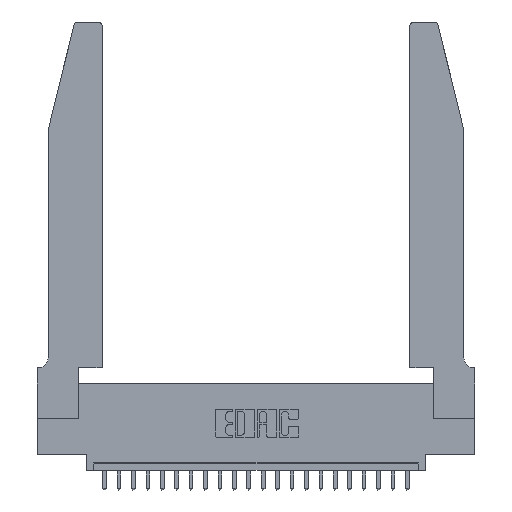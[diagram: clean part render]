
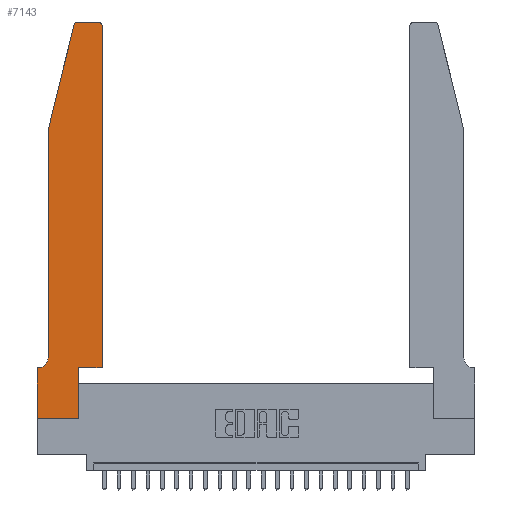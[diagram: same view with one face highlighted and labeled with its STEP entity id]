
A CAD part, top view. The second image highlights one B-rep face of the part: STEP entity #7143.
In plain terms, the highlighted planar face has unit normal (0, 0, 1).
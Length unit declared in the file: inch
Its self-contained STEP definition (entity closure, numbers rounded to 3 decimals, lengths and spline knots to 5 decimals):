
#293 = DIRECTION ( 'NONE',  ( -1., 0., 0. ) ) ;
#314 = FACE_OUTER_BOUND ( 'NONE', #9441, .T. ) ;
#505 = VECTOR ( 'NONE', #293, 39.37008 ) ;
#648 = LINE ( 'NONE', #7315, #7947 ) ;
#651 = EDGE_CURVE ( 'NONE', #10738, #8903, #2196, .T. ) ;
#888 = CARTESIAN_POINT ( 'NONE',  ( 0.2865, 0.35, 0.37 ) ) ;
#1593 = CARTESIAN_POINT ( 'NONE',  ( 0.25487, 2.72718, 0.37 ) ) ;
#1778 = DIRECTION ( 'NONE',  ( 0., 0., 1. ) ) ;
#1845 = VERTEX_POINT ( 'NONE', #3030 ) ;
#1966 = AXIS2_PLACEMENT_3D ( 'NONE', #5662, #3877, #18758 ) ;
#2196 = CIRCLE ( 'NONE', #1966, 0.03 ) ;
#2207 = VECTOR ( 'NONE', #19193, 39.37008 ) ;
#2214 = DIRECTION ( 'NONE',  ( -0.239, -0.971, 0. ) ) ;
#2424 = EDGE_CURVE ( 'NONE', #22252, #14683, #8212, .T. ) ;
#2864 = EDGE_CURVE ( 'NONE', #10535, #8425, #7298, .T. ) ;
#3030 = CARTESIAN_POINT ( 'NONE',  ( 0., 0., 0.37 ) ) ;
#3365 = ORIENTED_EDGE ( 'NONE', *, *, #17456, .T. ) ;
#3717 = DIRECTION ( 'NONE',  ( 0., 1., 0. ) ) ;
#3795 = CARTESIAN_POINT ( 'NONE',  ( 0.0755, 2., 0.37 ) ) ;
#3809 = DIRECTION ( 'NONE',  ( 1., 0., 0. ) ) ;
#3814 = CARTESIAN_POINT ( 'NONE',  ( 0.2865, 0.35, 0.37 ) ) ;
#3877 = DIRECTION ( 'NONE',  ( 0., 0., 1. ) ) ;
#4504 = VERTEX_POINT ( 'NONE', #6950 ) ;
#4551 = VECTOR ( 'NONE', #2214, 39.37008 ) ;
#4556 = CARTESIAN_POINT ( 'NONE',  ( 0.0755, 0.35, 0.37 ) ) ;
#5016 = CARTESIAN_POINT ( 'NONE',  ( 0.4505, 0.35, 0.37 ) ) ;
#5412 = AXIS2_PLACEMENT_3D ( 'NONE', #11856, #19323, #9997 ) ;
#5566 = DIRECTION ( 'NONE',  ( 1., 0., 0. ) ) ;
#5662 = CARTESIAN_POINT ( 'NONE',  ( 0.4205, 2.72, 0.37 ) ) ;
#5712 = CARTESIAN_POINT ( 'NONE',  ( 0.0755, 2., 0.37 ) ) ;
#5928 = LINE ( 'NONE', #9291, #23110 ) ;
#6068 = CARTESIAN_POINT ( 'NONE',  ( 0.0055, 0.35, 0.37 ) ) ;
#6135 = CARTESIAN_POINT ( 'NONE',  ( 0.284, 2.75, 0.37 ) ) ;
#6295 = DIRECTION ( 'NONE',  ( 1., 0., 0. ) ) ;
#6394 = ORIENTED_EDGE ( 'NONE', *, *, #24182, .T. ) ;
#6432 = ORIENTED_EDGE ( 'NONE', *, *, #651, .T. ) ;
#6544 = EDGE_CURVE ( 'NONE', #10442, #22252, #6596, .T. ) ;
#6596 = LINE ( 'NONE', #19973, #2207 ) ;
#6754 = VECTOR ( 'NONE', #6295, 39.37008 ) ;
#6950 = CARTESIAN_POINT ( 'NONE',  ( 0., 0.35, 0.37 ) ) ;
#7143 = ADVANCED_FACE ( 'NONE', ( #314 ), #22211, .T. ) ;
#7298 = CIRCLE ( 'NONE', #20075, 0.03 ) ;
#7315 = CARTESIAN_POINT ( 'NONE',  ( 0., 0., 0.37 ) ) ;
#7947 = VECTOR ( 'NONE', #10768, 39.37008 ) ;
#8212 = CIRCLE ( 'NONE', #5412, 0.07 ) ;
#8397 = CARTESIAN_POINT ( 'NONE',  ( 0.284, 2.72, 0.37 ) ) ;
#8425 = VERTEX_POINT ( 'NONE', #1593 ) ;
#8903 = VERTEX_POINT ( 'NONE', #15003 ) ;
#9291 = CARTESIAN_POINT ( 'NONE',  ( 0.4505, 0.35, 0.37 ) ) ;
#9441 = EDGE_LOOP ( 'NONE', ( #6394, #18322, #14975, #13087, #12427, #12759, #20394, #3365, #23756, #10246, #21108, #6432 ) ) ;
#9997 = DIRECTION ( 'NONE',  ( -1., 0., 0. ) ) ;
#10246 = ORIENTED_EDGE ( 'NONE', *, *, #15435, .T. ) ;
#10442 = VERTEX_POINT ( 'NONE', #3795 ) ;
#10535 = VERTEX_POINT ( 'NONE', #6135 ) ;
#10738 = VERTEX_POINT ( 'NONE', #23905 ) ;
#10768 = DIRECTION ( 'NONE',  ( 0., -1., 0. ) ) ;
#11157 = DIRECTION ( 'NONE',  ( 0., 1., 0. ) ) ;
#11558 = VECTOR ( 'NONE', #18023, 39.37008 ) ;
#11678 = LINE ( 'NONE', #3814, #21056 ) ;
#11856 = CARTESIAN_POINT ( 'NONE',  ( 0.0055, 0.42, 0.37 ) ) ;
#12201 = EDGE_CURVE ( 'NONE', #17819, #22700, #11678, .T. ) ;
#12427 = ORIENTED_EDGE ( 'NONE', *, *, #2424, .T. ) ;
#12623 = EDGE_CURVE ( 'NONE', #4504, #1845, #648, .T. ) ;
#12759 = ORIENTED_EDGE ( 'NONE', *, *, #20448, .T. ) ;
#12860 = EDGE_CURVE ( 'NONE', #22322, #10738, #5928, .T. ) ;
#12993 = LINE ( 'NONE', #13152, #505 ) ;
#13087 = ORIENTED_EDGE ( 'NONE', *, *, #6544, .T. ) ;
#13152 = CARTESIAN_POINT ( 'NONE',  ( 0.2605, 2.75, 0.37 ) ) ;
#14223 = LINE ( 'NONE', #22167, #11558 ) ;
#14683 = VERTEX_POINT ( 'NONE', #6068 ) ;
#14952 = LINE ( 'NONE', #5712, #4551 ) ;
#14975 = ORIENTED_EDGE ( 'NONE', *, *, #18838, .T. ) ;
#15003 = CARTESIAN_POINT ( 'NONE',  ( 0.4205, 2.75, 0.37 ) ) ;
#15435 = EDGE_CURVE ( 'NONE', #22700, #22322, #18653, .T. ) ;
#16725 = CARTESIAN_POINT ( 'NONE',  ( 0., 0.35, 0.37 ) ) ;
#17456 = EDGE_CURVE ( 'NONE', #1845, #17819, #14223, .T. ) ;
#17819 = VERTEX_POINT ( 'NONE', #19715 ) ;
#18023 = DIRECTION ( 'NONE',  ( 1., 0., 0. ) ) ;
#18322 = ORIENTED_EDGE ( 'NONE', *, *, #2864, .T. ) ;
#18653 = LINE ( 'NONE', #19383, #6754 ) ;
#18758 = DIRECTION ( 'NONE',  ( 1., 0., 0. ) ) ;
#18838 = EDGE_CURVE ( 'NONE', #8425, #10442, #14952, .T. ) ;
#19193 = DIRECTION ( 'NONE',  ( 0., -1., 0. ) ) ;
#19205 = DIRECTION ( 'NONE',  ( -1., 0., 0. ) ) ;
#19323 = DIRECTION ( 'NONE',  ( 0., 0., -1. ) ) ;
#19383 = CARTESIAN_POINT ( 'NONE',  ( 0.4505, 0.35, 0.37 ) ) ;
#19715 = CARTESIAN_POINT ( 'NONE',  ( 0.2865, 0., 0.37 ) ) ;
#19748 = CARTESIAN_POINT ( 'NONE',  ( 0.0755, 0.42, 0.37 ) ) ;
#19829 = DIRECTION ( 'NONE',  ( 0., 0., 1. ) ) ;
#19973 = CARTESIAN_POINT ( 'NONE',  ( 0.0755, 2., 0.37 ) ) ;
#20075 = AXIS2_PLACEMENT_3D ( 'NONE', #8397, #19829, #5566 ) ;
#20394 = ORIENTED_EDGE ( 'NONE', *, *, #12623, .T. ) ;
#20448 = EDGE_CURVE ( 'NONE', #14683, #4504, #22900, .T. ) ;
#21056 = VECTOR ( 'NONE', #3717, 39.37008 ) ;
#21108 = ORIENTED_EDGE ( 'NONE', *, *, #12860, .T. ) ;
#21130 = VECTOR ( 'NONE', #19205, 39.37008 ) ;
#22167 = CARTESIAN_POINT ( 'NONE',  ( 0., 0., 0.37 ) ) ;
#22211 = PLANE ( 'NONE',  #22965 ) ;
#22252 = VERTEX_POINT ( 'NONE', #19748 ) ;
#22322 = VERTEX_POINT ( 'NONE', #5016 ) ;
#22700 = VERTEX_POINT ( 'NONE', #888 ) ;
#22900 = LINE ( 'NONE', #4556, #21130 ) ;
#22965 = AXIS2_PLACEMENT_3D ( 'NONE', #16725, #1778, #3809 ) ;
#23110 = VECTOR ( 'NONE', #11157, 39.37008 ) ;
#23756 = ORIENTED_EDGE ( 'NONE', *, *, #12201, .T. ) ;
#23905 = CARTESIAN_POINT ( 'NONE',  ( 0.4505, 2.72, 0.37 ) ) ;
#24182 = EDGE_CURVE ( 'NONE', #8903, #10535, #12993, .T. ) ;
